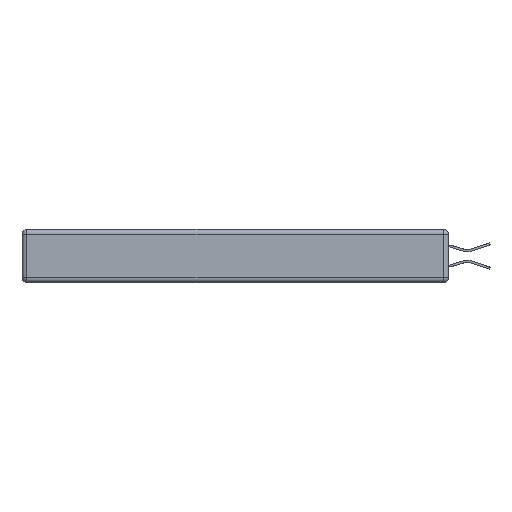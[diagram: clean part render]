
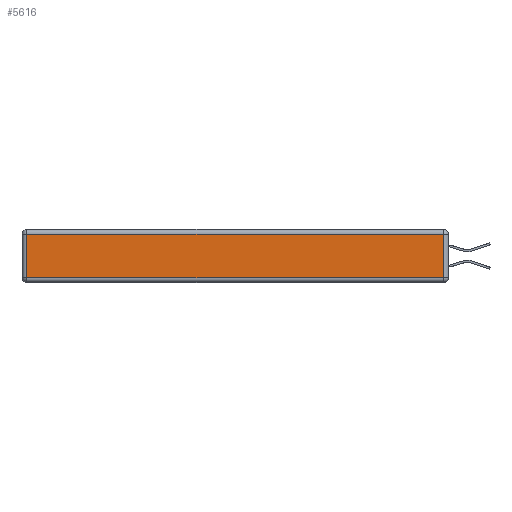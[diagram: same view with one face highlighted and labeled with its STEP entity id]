
A CAD part, left-side view. The second image highlights one B-rep face of the part: STEP entity #5616.
In plain terms, the highlighted planar face has unit normal (-1, 0, 0).
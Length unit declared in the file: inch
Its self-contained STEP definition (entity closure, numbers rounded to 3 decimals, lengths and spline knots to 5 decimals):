
#155 = CARTESIAN_POINT ( 'NONE',  ( 0., 0.03, -0.343 ) ) ;
#666 = LINE ( 'NONE', #13758, #6369 ) ;
#877 = CARTESIAN_POINT ( 'NONE',  ( 0., 0.03, -0.03 ) ) ;
#993 = VERTEX_POINT ( 'NONE', #877 ) ;
#1237 = ORIENTED_EDGE ( 'NONE', *, *, #3486, .T. ) ;
#1783 = DIRECTION ( 'NONE',  ( -1., 0., 0. ) ) ;
#1902 = DIRECTION ( 'NONE',  ( 0., 0., 1. ) ) ;
#3325 = ORIENTED_EDGE ( 'NONE', *, *, #7932, .T. ) ;
#3486 = EDGE_CURVE ( 'NONE', #10907, #993, #6660, .T. ) ;
#3753 = CARTESIAN_POINT ( 'NONE',  ( 0., 2.72, -0.343 ) ) ;
#4522 = CARTESIAN_POINT ( 'NONE',  ( 0., 0.03, -0.313 ) ) ;
#5136 = EDGE_CURVE ( 'NONE', #993, #13256, #14475, .T. ) ;
#5509 = DIRECTION ( 'NONE',  ( 0., 1., 0. ) ) ;
#5616 = ADVANCED_FACE ( 'NONE', ( #10560 ), #7378, .T. ) ;
#6211 = VECTOR ( 'NONE', #9988, 39.37008 ) ;
#6369 = VECTOR ( 'NONE', #13580, 39.37008 ) ;
#6660 = LINE ( 'NONE', #155, #6211 ) ;
#7230 = LINE ( 'NONE', #3753, #17675 ) ;
#7378 = PLANE ( 'NONE',  #8970 ) ;
#7435 = CARTESIAN_POINT ( 'NONE',  ( 0., 0., -0.343 ) ) ;
#7789 = VERTEX_POINT ( 'NONE', #17770 ) ;
#7849 = ORIENTED_EDGE ( 'NONE', *, *, #5136, .T. ) ;
#7932 = EDGE_CURVE ( 'NONE', #7789, #10907, #666, .T. ) ;
#8839 = EDGE_CURVE ( 'NONE', #13256, #7789, #7230, .T. ) ;
#8970 = AXIS2_PLACEMENT_3D ( 'NONE', #7435, #1783, #1902 ) ;
#9538 = CARTESIAN_POINT ( 'NONE',  ( 0., 2.72, -0.03 ) ) ;
#9988 = DIRECTION ( 'NONE',  ( 0., 0., 1. ) ) ;
#10560 = FACE_OUTER_BOUND ( 'NONE', #14484, .T. ) ;
#10907 = VERTEX_POINT ( 'NONE', #4522 ) ;
#11688 = ORIENTED_EDGE ( 'NONE', *, *, #8839, .T. ) ;
#13256 = VERTEX_POINT ( 'NONE', #9538 ) ;
#13558 = DIRECTION ( 'NONE',  ( 0., 0., -1. ) ) ;
#13580 = DIRECTION ( 'NONE',  ( 0., -1., 0. ) ) ;
#13758 = CARTESIAN_POINT ( 'NONE',  ( 0., 0., -0.313 ) ) ;
#13823 = CARTESIAN_POINT ( 'NONE',  ( 0., 2.75, -0.03 ) ) ;
#14475 = LINE ( 'NONE', #13823, #17534 ) ;
#14484 = EDGE_LOOP ( 'NONE', ( #3325, #1237, #7849, #11688 ) ) ;
#17534 = VECTOR ( 'NONE', #5509, 39.37008 ) ;
#17675 = VECTOR ( 'NONE', #13558, 39.37008 ) ;
#17770 = CARTESIAN_POINT ( 'NONE',  ( 0., 2.72, -0.313 ) ) ;
